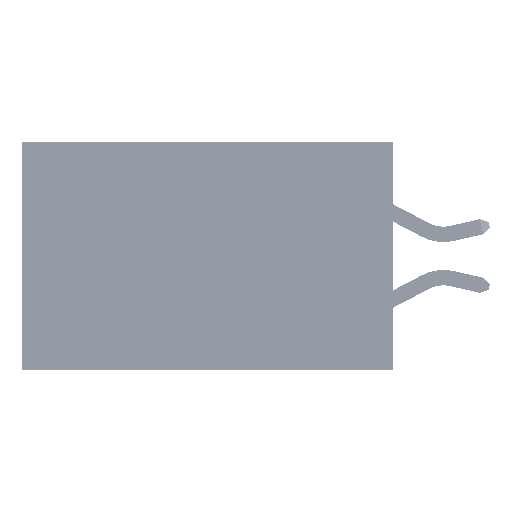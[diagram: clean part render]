
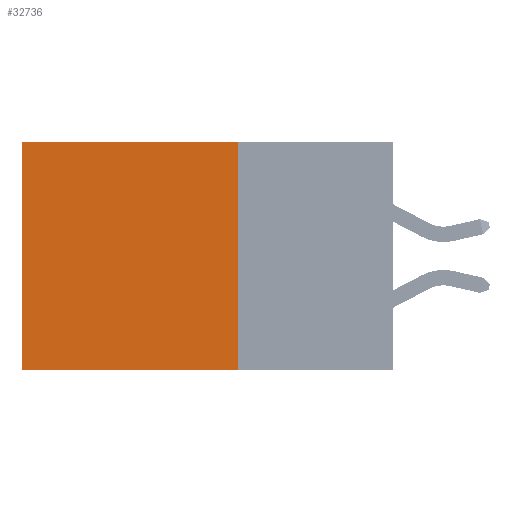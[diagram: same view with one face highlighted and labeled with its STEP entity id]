
A CAD part, left-side view. The second image highlights one B-rep face of the part: STEP entity #32736.
In plain terms, the highlighted planar face has unit normal (-1, 0, 0).
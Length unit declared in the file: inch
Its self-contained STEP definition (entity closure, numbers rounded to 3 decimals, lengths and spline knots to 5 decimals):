
#18 = CARTESIAN_POINT ( 'NONE',  ( 0.2875, 0.25, -0.37 ) ) ;
#6789 = VERTEX_POINT ( 'NONE', #12251 ) ;
#7634 = VERTEX_POINT ( 'NONE', #16432 ) ;
#8628 = CARTESIAN_POINT ( 'NONE',  ( 0.2875, 0.6, -0.37 ) ) ;
#11380 = EDGE_CURVE ( 'NONE', #7634, #34835, #27784, .T. ) ;
#11946 = EDGE_CURVE ( 'NONE', #40820, #6789, #22600, .T. ) ;
#12251 = CARTESIAN_POINT ( 'NONE',  ( 0.2875, 0.25, -0.37 ) ) ;
#14696 = AXIS2_PLACEMENT_3D ( 'NONE', #41130, #28946, #45012 ) ;
#15095 = FACE_OUTER_BOUND ( 'NONE', #50976, .T. ) ;
#16432 = CARTESIAN_POINT ( 'NONE',  ( 0.2875, 0.6, 0. ) ) ;
#16693 = PLANE ( 'NONE',  #14696 ) ;
#20739 = VECTOR ( 'NONE', #48127, 39.37008 ) ;
#21328 = VECTOR ( 'NONE', #48155, 39.37008 ) ;
#21694 = EDGE_CURVE ( 'NONE', #6789, #34835, #36085, .T. ) ;
#22479 = ORIENTED_EDGE ( 'NONE', *, *, #31014, .T. ) ;
#22600 = LINE ( 'NONE', #51888, #21328 ) ;
#24157 = CARTESIAN_POINT ( 'NONE',  ( 0.2875, 0.6, 0. ) ) ;
#25438 = LINE ( 'NONE', #42910, #42707 ) ;
#27784 = LINE ( 'NONE', #24157, #51384 ) ;
#28946 = DIRECTION ( 'NONE',  ( 1., 0., 0. ) ) ;
#30428 = DIRECTION ( 'NONE',  ( 0., 1., 0. ) ) ;
#31014 = EDGE_CURVE ( 'NONE', #40820, #7634, #25438, .T. ) ;
#32736 = ADVANCED_FACE ( 'NONE', ( #15095 ), #16693, .F. ) ;
#34835 = VERTEX_POINT ( 'NONE', #8628 ) ;
#36085 = LINE ( 'NONE', #18, #20739 ) ;
#40281 = CARTESIAN_POINT ( 'NONE',  ( 0.2875, 0.25, 0. ) ) ;
#40820 = VERTEX_POINT ( 'NONE', #40281 ) ;
#41130 = CARTESIAN_POINT ( 'NONE',  ( 0.2875, 0.25, 0. ) ) ;
#42707 = VECTOR ( 'NONE', #30428, 39.37008 ) ;
#42910 = CARTESIAN_POINT ( 'NONE',  ( 0.2875, 0.25, 0. ) ) ;
#44556 = ORIENTED_EDGE ( 'NONE', *, *, #11946, .F. ) ;
#45012 = DIRECTION ( 'NONE',  ( 0., 0., -1. ) ) ;
#46714 = ORIENTED_EDGE ( 'NONE', *, *, #21694, .F. ) ;
#48127 = DIRECTION ( 'NONE',  ( 0., 1., 0. ) ) ;
#48155 = DIRECTION ( 'NONE',  ( 0., 0., -1. ) ) ;
#49295 = DIRECTION ( 'NONE',  ( 0., 0., -1. ) ) ;
#50976 = EDGE_LOOP ( 'NONE', ( #51474, #46714, #44556, #22479 ) ) ;
#51384 = VECTOR ( 'NONE', #49295, 39.37008 ) ;
#51474 = ORIENTED_EDGE ( 'NONE', *, *, #11380, .T. ) ;
#51888 = CARTESIAN_POINT ( 'NONE',  ( 0.2875, 0.25, 0. ) ) ;
